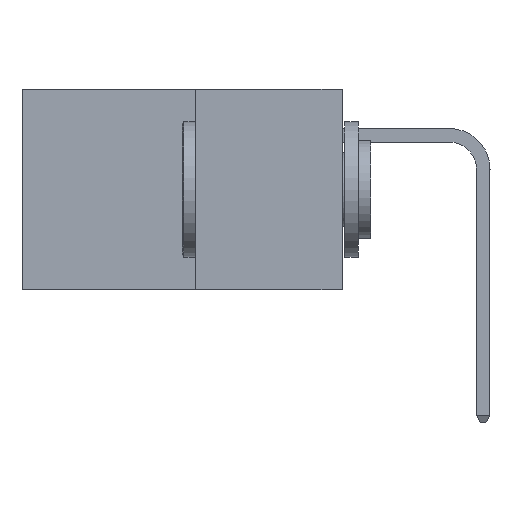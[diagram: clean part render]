
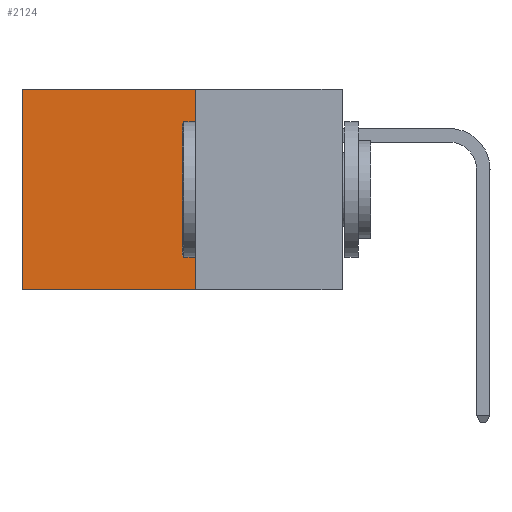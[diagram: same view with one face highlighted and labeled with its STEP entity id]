
A CAD part, left-side view. The second image highlights one B-rep face of the part: STEP entity #2124.
In plain terms, the highlighted planar face has unit normal (-1, 0, 0).
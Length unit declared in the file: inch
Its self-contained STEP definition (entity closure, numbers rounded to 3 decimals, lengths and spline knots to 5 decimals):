
#380 = LINE ( 'NONE', #8330, #12619 ) ;
#410 = CARTESIAN_POINT ( 'NONE',  ( 0.277, 0.27, -0.37 ) ) ;
#575 = EDGE_CURVE ( 'NONE', #2367, #12982, #380, .T. ) ;
#990 = AXIS2_PLACEMENT_3D ( 'NONE', #410, #8431, #1075 ) ;
#1075 = DIRECTION ( 'NONE',  ( 0., 0., -1. ) ) ;
#1233 = CARTESIAN_POINT ( 'NONE',  ( 0.277, 0.27, 0. ) ) ;
#1625 = CARTESIAN_POINT ( 'NONE',  ( 0.277, 0.27, 0. ) ) ;
#1844 = EDGE_CURVE ( 'NONE', #10480, #10195, #9449, .T. ) ;
#2124 = ADVANCED_FACE ( 'NONE', ( #5092 ), #8983, .F. ) ;
#2367 = VERTEX_POINT ( 'NONE', #8865 ) ;
#2870 = ORIENTED_EDGE ( 'NONE', *, *, #14892, .T. ) ;
#3437 = DIRECTION ( 'NONE',  ( 0., 0., -1. ) ) ;
#3746 = ORIENTED_EDGE ( 'NONE', *, *, #1844, .F. ) ;
#3787 = EDGE_CURVE ( 'NONE', #10195, #12982, #11338, .T. ) ;
#4728 = CARTESIAN_POINT ( 'NONE',  ( 0.277, 0.27, -0.37 ) ) ;
#5092 = FACE_OUTER_BOUND ( 'NONE', #12049, .T. ) ;
#5148 = DIRECTION ( 'NONE',  ( 0., 0., -1. ) ) ;
#5294 = CARTESIAN_POINT ( 'NONE',  ( 0.277, 0.59, -0.37 ) ) ;
#5376 = ORIENTED_EDGE ( 'NONE', *, *, #3787, .F. ) ;
#6054 = VECTOR ( 'NONE', #3437, 39.37008 ) ;
#6248 = VECTOR ( 'NONE', #14159, 39.37008 ) ;
#7264 = DIRECTION ( 'NONE',  ( 0., 1., 0. ) ) ;
#8191 = CARTESIAN_POINT ( 'NONE',  ( 0.277, 0.27, -0.37 ) ) ;
#8330 = CARTESIAN_POINT ( 'NONE',  ( 0.277, 0.59, -0.37 ) ) ;
#8360 = CARTESIAN_POINT ( 'NONE',  ( 0.277, 0.27, -0.37 ) ) ;
#8431 = DIRECTION ( 'NONE',  ( 1., 0., 0. ) ) ;
#8803 = ORIENTED_EDGE ( 'NONE', *, *, #575, .T. ) ;
#8865 = CARTESIAN_POINT ( 'NONE',  ( 0.277, 0.59, 0. ) ) ;
#8983 = PLANE ( 'NONE',  #990 ) ;
#9449 = LINE ( 'NONE', #4728, #6054 ) ;
#10195 = VERTEX_POINT ( 'NONE', #8360 ) ;
#10480 = VERTEX_POINT ( 'NONE', #1625 ) ;
#10976 = VECTOR ( 'NONE', #7264, 39.37008 ) ;
#11338 = LINE ( 'NONE', #8191, #10976 ) ;
#12049 = EDGE_LOOP ( 'NONE', ( #8803, #5376, #3746, #2870 ) ) ;
#12619 = VECTOR ( 'NONE', #5148, 39.37008 ) ;
#12982 = VERTEX_POINT ( 'NONE', #5294 ) ;
#14159 = DIRECTION ( 'NONE',  ( 0., 1., 0. ) ) ;
#14892 = EDGE_CURVE ( 'NONE', #10480, #2367, #15181, .T. ) ;
#15181 = LINE ( 'NONE', #1233, #6248 ) ;
